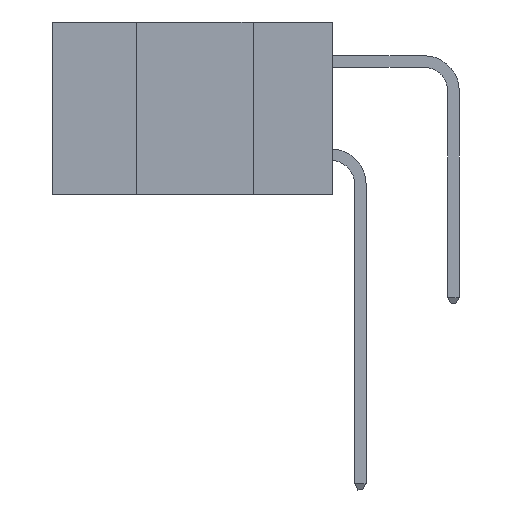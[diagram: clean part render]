
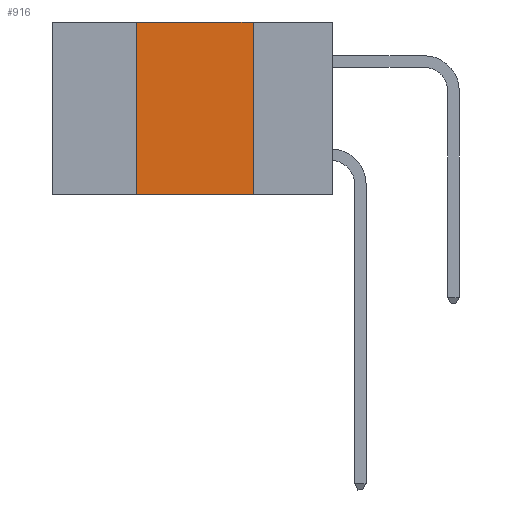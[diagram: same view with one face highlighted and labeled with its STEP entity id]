
A CAD part, left-side view. The second image highlights one B-rep face of the part: STEP entity #916.
In plain terms, the highlighted planar face has unit normal (-1, 0, 0).
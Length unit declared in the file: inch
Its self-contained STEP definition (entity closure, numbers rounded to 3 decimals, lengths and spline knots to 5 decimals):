
#602 = DIRECTION ( 'NONE',  ( 0., -1., 0. ) ) ;
#889 = VECTOR ( 'NONE', #19944, 39.37008 ) ;
#916 = ADVANCED_FACE ( 'NONE', ( #2979 ), #22897, .F. ) ;
#2979 = FACE_OUTER_BOUND ( 'NONE', #23971, .T. ) ;
#3870 = CARTESIAN_POINT ( 'NONE',  ( 0., 0.17, -0.37 ) ) ;
#6656 = CARTESIAN_POINT ( 'NONE',  ( 0., 0.6, 0. ) ) ;
#8786 = EDGE_CURVE ( 'NONE', #28290, #26821, #28076, .T. ) ;
#9437 = DIRECTION ( 'NONE',  ( 0., -1., 0. ) ) ;
#9876 = LINE ( 'NONE', #27958, #27291 ) ;
#11758 = CARTESIAN_POINT ( 'NONE',  ( 0., 0.6, 0. ) ) ;
#12103 = CARTESIAN_POINT ( 'NONE',  ( 0., 0.42, -0.37 ) ) ;
#12467 = ORIENTED_EDGE ( 'NONE', *, *, #15489, .F. ) ;
#14170 = VECTOR ( 'NONE', #9437, 39.37008 ) ;
#14361 = CARTESIAN_POINT ( 'NONE',  ( 0., 0.42, -0.37 ) ) ;
#15489 = EDGE_CURVE ( 'NONE', #19409, #17872, #24539, .T. ) ;
#16663 = DIRECTION ( 'NONE',  ( 0., 0., 1. ) ) ;
#16905 = DIRECTION ( 'NONE',  ( 1., 0., 0. ) ) ;
#17163 = ORIENTED_EDGE ( 'NONE', *, *, #8786, .F. ) ;
#17446 = EDGE_CURVE ( 'NONE', #26821, #19409, #23037, .T. ) ;
#17872 = VERTEX_POINT ( 'NONE', #19987 ) ;
#19409 = VERTEX_POINT ( 'NONE', #20498 ) ;
#19944 = DIRECTION ( 'NONE',  ( 0., 0., -1. ) ) ;
#19987 = CARTESIAN_POINT ( 'NONE',  ( 0., 0.17, -0.37 ) ) ;
#20498 = CARTESIAN_POINT ( 'NONE',  ( 0., 0.17, 0. ) ) ;
#22134 = VECTOR ( 'NONE', #16663, 39.37008 ) ;
#22897 = PLANE ( 'NONE',  #23862 ) ;
#23037 = LINE ( 'NONE', #11758, #14170 ) ;
#23656 = EDGE_CURVE ( 'NONE', #28290, #17872, #9876, .T. ) ;
#23862 = AXIS2_PLACEMENT_3D ( 'NONE', #6656, #16905, #29026 ) ;
#23971 = EDGE_LOOP ( 'NONE', ( #12467, #25262, #17163, #27530 ) ) ;
#24539 = LINE ( 'NONE', #3870, #889 ) ;
#25262 = ORIENTED_EDGE ( 'NONE', *, *, #17446, .F. ) ;
#26821 = VERTEX_POINT ( 'NONE', #26847 ) ;
#26847 = CARTESIAN_POINT ( 'NONE',  ( 0., 0.42, 0. ) ) ;
#27291 = VECTOR ( 'NONE', #602, 39.37008 ) ;
#27530 = ORIENTED_EDGE ( 'NONE', *, *, #23656, .T. ) ;
#27958 = CARTESIAN_POINT ( 'NONE',  ( 0., 0.6, -0.37 ) ) ;
#28076 = LINE ( 'NONE', #14361, #22134 ) ;
#28290 = VERTEX_POINT ( 'NONE', #12103 ) ;
#29026 = DIRECTION ( 'NONE',  ( 0., 0., -1. ) ) ;
